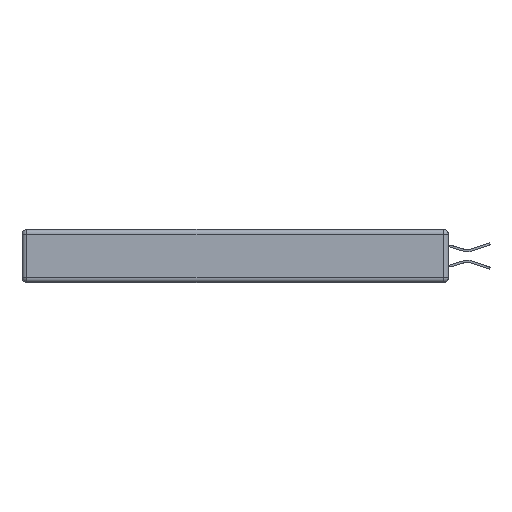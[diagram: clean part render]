
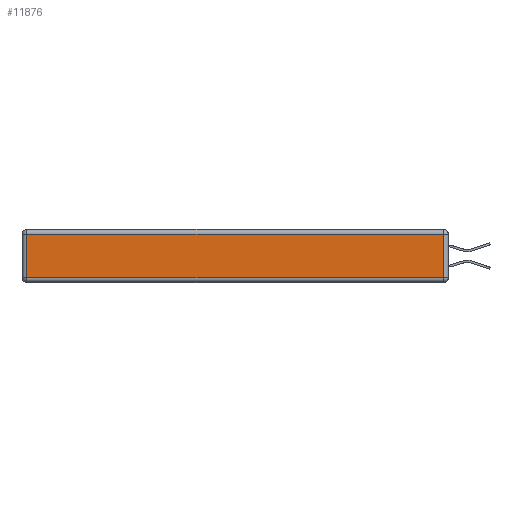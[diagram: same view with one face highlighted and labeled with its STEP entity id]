
A CAD part, left-side view. The second image highlights one B-rep face of the part: STEP entity #11876.
In plain terms, the highlighted planar face has unit normal (-1, 0, 0).
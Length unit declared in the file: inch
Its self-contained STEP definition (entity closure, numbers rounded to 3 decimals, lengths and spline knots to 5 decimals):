
#1410 = ORIENTED_EDGE ( 'NONE', *, *, #6743, .T. ) ;
#1576 = ORIENTED_EDGE ( 'NONE', *, *, #6320, .T. ) ;
#1606 = LINE ( 'NONE', #4025, #21810 ) ;
#1882 = DIRECTION ( 'NONE',  ( 0., 0., -1. ) ) ;
#2184 = LINE ( 'NONE', #21369, #3595 ) ;
#3595 = VECTOR ( 'NONE', #1882, 39.37008 ) ;
#3795 = DIRECTION ( 'NONE',  ( 0., 0., 1. ) ) ;
#4025 = CARTESIAN_POINT ( 'NONE',  ( 0., 0.03, -0.343 ) ) ;
#5015 = CARTESIAN_POINT ( 'NONE',  ( 0., 0., -0.343 ) ) ;
#6160 = ORIENTED_EDGE ( 'NONE', *, *, #21602, .T. ) ;
#6320 = EDGE_CURVE ( 'NONE', #21107, #11519, #12702, .T. ) ;
#6743 = EDGE_CURVE ( 'NONE', #11519, #8707, #1606, .T. ) ;
#7614 = CARTESIAN_POINT ( 'NONE',  ( 0., 0.03, -0.313 ) ) ;
#7742 = VECTOR ( 'NONE', #9120, 39.37008 ) ;
#8707 = VERTEX_POINT ( 'NONE', #14689 ) ;
#9065 = ORIENTED_EDGE ( 'NONE', *, *, #20172, .T. ) ;
#9120 = DIRECTION ( 'NONE',  ( 0., -1., 0. ) ) ;
#9274 = CARTESIAN_POINT ( 'NONE',  ( 0., 0., -0.313 ) ) ;
#9391 = CARTESIAN_POINT ( 'NONE',  ( 0., 2.72, -0.03 ) ) ;
#9479 = VECTOR ( 'NONE', #9710, 39.37008 ) ;
#9710 = DIRECTION ( 'NONE',  ( 0., 1., 0. ) ) ;
#11519 = VERTEX_POINT ( 'NONE', #7614 ) ;
#11538 = VERTEX_POINT ( 'NONE', #9391 ) ;
#11876 = ADVANCED_FACE ( 'NONE', ( #19631 ), #15622, .T. ) ;
#12702 = LINE ( 'NONE', #9274, #7742 ) ;
#14147 = DIRECTION ( 'NONE',  ( -1., 0., 0. ) ) ;
#14166 = LINE ( 'NONE', #17952, #9479 ) ;
#14689 = CARTESIAN_POINT ( 'NONE',  ( 0., 0.03, -0.03 ) ) ;
#15622 = PLANE ( 'NONE',  #19622 ) ;
#17952 = CARTESIAN_POINT ( 'NONE',  ( 0., 2.75, -0.03 ) ) ;
#18122 = CARTESIAN_POINT ( 'NONE',  ( 0., 2.72, -0.313 ) ) ;
#19622 = AXIS2_PLACEMENT_3D ( 'NONE', #5015, #14147, #20873 ) ;
#19631 = FACE_OUTER_BOUND ( 'NONE', #21509, .T. ) ;
#20172 = EDGE_CURVE ( 'NONE', #8707, #11538, #14166, .T. ) ;
#20873 = DIRECTION ( 'NONE',  ( 0., 0., 1. ) ) ;
#21107 = VERTEX_POINT ( 'NONE', #18122 ) ;
#21369 = CARTESIAN_POINT ( 'NONE',  ( 0., 2.72, -0.343 ) ) ;
#21509 = EDGE_LOOP ( 'NONE', ( #1576, #1410, #9065, #6160 ) ) ;
#21602 = EDGE_CURVE ( 'NONE', #11538, #21107, #2184, .T. ) ;
#21810 = VECTOR ( 'NONE', #3795, 39.37008 ) ;
